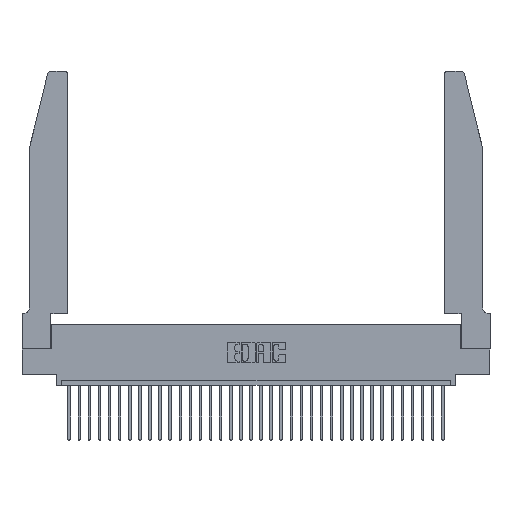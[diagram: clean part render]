
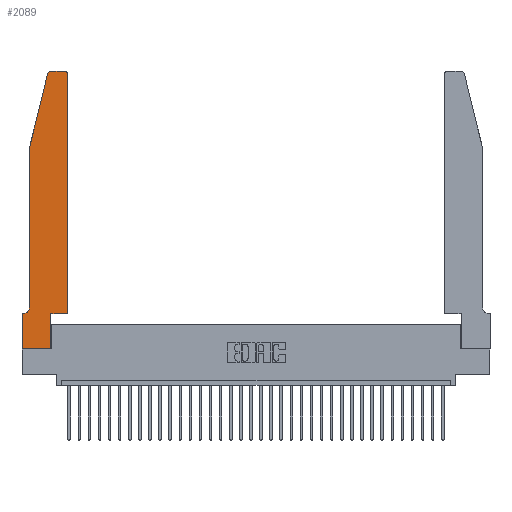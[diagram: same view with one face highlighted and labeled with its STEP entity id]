
A CAD part, top view. The second image highlights one B-rep face of the part: STEP entity #2089.
In plain terms, the highlighted planar face has unit normal (0, 0, 1).
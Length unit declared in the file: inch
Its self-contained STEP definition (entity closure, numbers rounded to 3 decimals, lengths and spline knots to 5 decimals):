
#426 = EDGE_CURVE ( 'NONE', #19606, #13271, #20745, .T. ) ;
#628 = LINE ( 'NONE', #29261, #20833 ) ;
#988 = ORIENTED_EDGE ( 'NONE', *, *, #8348, .T. ) ;
#1811 = ORIENTED_EDGE ( 'NONE', *, *, #30417, .T. ) ;
#2089 = ADVANCED_FACE ( 'NONE', ( #4976 ), #28690, .T. ) ;
#2263 = CARTESIAN_POINT ( 'NONE',  ( 0.4205, 2.75, 0.37 ) ) ;
#2933 = EDGE_CURVE ( 'NONE', #13580, #11461, #31247, .T. ) ;
#3570 = DIRECTION ( 'NONE',  ( 1., 0., 0. ) ) ;
#3638 = ORIENTED_EDGE ( 'NONE', *, *, #2933, .T. ) ;
#4335 = VECTOR ( 'NONE', #23577, 39.37008 ) ;
#4351 = CARTESIAN_POINT ( 'NONE',  ( 0.0755, 2., 0.37 ) ) ;
#4896 = CARTESIAN_POINT ( 'NONE',  ( 0.4205, 2.72, 0.37 ) ) ;
#4976 = FACE_OUTER_BOUND ( 'NONE', #11247, .T. ) ;
#5119 = CARTESIAN_POINT ( 'NONE',  ( 0., 0., 0.37 ) ) ;
#5336 = VECTOR ( 'NONE', #19750, 39.37008 ) ;
#5422 = CARTESIAN_POINT ( 'NONE',  ( 0.284, 2.75, 0.37 ) ) ;
#5726 = VECTOR ( 'NONE', #32244, 39.37008 ) ;
#6444 = CIRCLE ( 'NONE', #33436, 0.07 ) ;
#6450 = EDGE_CURVE ( 'NONE', #32554, #13580, #16539, .T. ) ;
#6557 = LINE ( 'NONE', #13905, #5726 ) ;
#6615 = CARTESIAN_POINT ( 'NONE',  ( 0.0755, 0.42, 0.37 ) ) ;
#7025 = ORIENTED_EDGE ( 'NONE', *, *, #426, .T. ) ;
#7287 = VECTOR ( 'NONE', #32134, 39.37008 ) ;
#7345 = VERTEX_POINT ( 'NONE', #21236 ) ;
#7951 = VERTEX_POINT ( 'NONE', #16158 ) ;
#8083 = EDGE_CURVE ( 'NONE', #18744, #15308, #19302, .T. ) ;
#8348 = EDGE_CURVE ( 'NONE', #11461, #10009, #6557, .T. ) ;
#8799 = CARTESIAN_POINT ( 'NONE',  ( 0., 0., 0.37 ) ) ;
#8819 = ORIENTED_EDGE ( 'NONE', *, *, #29166, .T. ) ;
#8914 = LINE ( 'NONE', #32735, #27896 ) ;
#8915 = CARTESIAN_POINT ( 'NONE',  ( 0., 0., 0.37 ) ) ;
#10009 = VERTEX_POINT ( 'NONE', #6615 ) ;
#10417 = DIRECTION ( 'NONE',  ( -1., 0., 0. ) ) ;
#11015 = VERTEX_POINT ( 'NONE', #5119 ) ;
#11247 = EDGE_LOOP ( 'NONE', ( #8819, #28361, #3638, #988, #25661, #15329, #26457, #33252, #12943, #1811, #26274, #7025 ) ) ;
#11461 = VERTEX_POINT ( 'NONE', #31204 ) ;
#12263 = LINE ( 'NONE', #33175, #17594 ) ;
#12943 = ORIENTED_EDGE ( 'NONE', *, *, #8083, .T. ) ;
#13071 = DIRECTION ( 'NONE',  ( 0., 0., -1. ) ) ;
#13271 = VERTEX_POINT ( 'NONE', #2263 ) ;
#13491 = DIRECTION ( 'NONE',  ( 0., 0., 1. ) ) ;
#13580 = VERTEX_POINT ( 'NONE', #24719 ) ;
#13905 = CARTESIAN_POINT ( 'NONE',  ( 0.0755, 2., 0.37 ) ) ;
#14028 = DIRECTION ( 'NONE',  ( 0., 1., 0. ) ) ;
#14168 = CARTESIAN_POINT ( 'NONE',  ( 0.284, 2.72, 0.37 ) ) ;
#14290 = LINE ( 'NONE', #8799, #7287 ) ;
#15308 = VERTEX_POINT ( 'NONE', #16961 ) ;
#15329 = ORIENTED_EDGE ( 'NONE', *, *, #16720, .T. ) ;
#15502 = DIRECTION ( 'NONE',  ( 1., 0., 0. ) ) ;
#16000 = EDGE_CURVE ( 'NONE', #25353, #11015, #14290, .T. ) ;
#16158 = CARTESIAN_POINT ( 'NONE',  ( 0.0055, 0.35, 0.37 ) ) ;
#16539 = CIRCLE ( 'NONE', #26204, 0.03 ) ;
#16720 = EDGE_CURVE ( 'NONE', #7951, #25353, #628, .T. ) ;
#16961 = CARTESIAN_POINT ( 'NONE',  ( 0.2865, 0.35, 0.37 ) ) ;
#17137 = CARTESIAN_POINT ( 'NONE',  ( 0.2865, 0., 0.37 ) ) ;
#17349 = DIRECTION ( 'NONE',  ( -0.239, -0.971, 0. ) ) ;
#17594 = VECTOR ( 'NONE', #25150, 39.37008 ) ;
#18253 = CARTESIAN_POINT ( 'NONE',  ( 0.0055, 0.42, 0.37 ) ) ;
#18405 = VECTOR ( 'NONE', #29961, 39.37008 ) ;
#18744 = VERTEX_POINT ( 'NONE', #17137 ) ;
#19290 = VECTOR ( 'NONE', #17349, 39.37008 ) ;
#19302 = LINE ( 'NONE', #19627, #5336 ) ;
#19606 = VERTEX_POINT ( 'NONE', #22176 ) ;
#19627 = CARTESIAN_POINT ( 'NONE',  ( 0.2865, 0.35, 0.37 ) ) ;
#19750 = DIRECTION ( 'NONE',  ( 0., 1., 0. ) ) ;
#20395 = EDGE_CURVE ( 'NONE', #7345, #19606, #8914, .T. ) ;
#20745 = CIRCLE ( 'NONE', #29779, 0.03 ) ;
#20833 = VECTOR ( 'NONE', #22249, 39.37008 ) ;
#21236 = CARTESIAN_POINT ( 'NONE',  ( 0.4505, 0.35, 0.37 ) ) ;
#22176 = CARTESIAN_POINT ( 'NONE',  ( 0.4505, 2.72, 0.37 ) ) ;
#22249 = DIRECTION ( 'NONE',  ( -1., 0., 0. ) ) ;
#23577 = DIRECTION ( 'NONE',  ( 1., 0., 0. ) ) ;
#24112 = CARTESIAN_POINT ( 'NONE',  ( 0., 0.35, 0.37 ) ) ;
#24719 = CARTESIAN_POINT ( 'NONE',  ( 0.25487, 2.72718, 0.37 ) ) ;
#25150 = DIRECTION ( 'NONE',  ( -1., 0., 0. ) ) ;
#25353 = VERTEX_POINT ( 'NONE', #24112 ) ;
#25661 = ORIENTED_EDGE ( 'NONE', *, *, #29189, .T. ) ;
#26204 = AXIS2_PLACEMENT_3D ( 'NONE', #14168, #27505, #3570 ) ;
#26274 = ORIENTED_EDGE ( 'NONE', *, *, #20395, .T. ) ;
#26457 = ORIENTED_EDGE ( 'NONE', *, *, #16000, .T. ) ;
#27505 = DIRECTION ( 'NONE',  ( 0., 0., 1. ) ) ;
#27896 = VECTOR ( 'NONE', #14028, 39.37008 ) ;
#28354 = DIRECTION ( 'NONE',  ( 0., 0., 1. ) ) ;
#28361 = ORIENTED_EDGE ( 'NONE', *, *, #6450, .T. ) ;
#28468 = CARTESIAN_POINT ( 'NONE',  ( 0., 0.35, 0.37 ) ) ;
#28499 = AXIS2_PLACEMENT_3D ( 'NONE', #28468, #28354, #15502 ) ;
#28690 = PLANE ( 'NONE',  #28499 ) ;
#28970 = EDGE_CURVE ( 'NONE', #11015, #18744, #32767, .T. ) ;
#29166 = EDGE_CURVE ( 'NONE', #13271, #32554, #12263, .T. ) ;
#29189 = EDGE_CURVE ( 'NONE', #10009, #7951, #6444, .T. ) ;
#29261 = CARTESIAN_POINT ( 'NONE',  ( 0.0755, 0.35, 0.37 ) ) ;
#29779 = AXIS2_PLACEMENT_3D ( 'NONE', #4896, #13491, #31845 ) ;
#29961 = DIRECTION ( 'NONE',  ( 1., 0., 0. ) ) ;
#30417 = EDGE_CURVE ( 'NONE', #15308, #7345, #30648, .T. ) ;
#30648 = LINE ( 'NONE', #33996, #4335 ) ;
#31204 = CARTESIAN_POINT ( 'NONE',  ( 0.0755, 2., 0.37 ) ) ;
#31247 = LINE ( 'NONE', #4351, #19290 ) ;
#31845 = DIRECTION ( 'NONE',  ( 1., 0., 0. ) ) ;
#32134 = DIRECTION ( 'NONE',  ( 0., -1., 0. ) ) ;
#32244 = DIRECTION ( 'NONE',  ( 0., -1., 0. ) ) ;
#32554 = VERTEX_POINT ( 'NONE', #5422 ) ;
#32735 = CARTESIAN_POINT ( 'NONE',  ( 0.4505, 0.35, 0.37 ) ) ;
#32767 = LINE ( 'NONE', #8915, #18405 ) ;
#33175 = CARTESIAN_POINT ( 'NONE',  ( 0.2605, 2.75, 0.37 ) ) ;
#33252 = ORIENTED_EDGE ( 'NONE', *, *, #28970, .T. ) ;
#33436 = AXIS2_PLACEMENT_3D ( 'NONE', #18253, #13071, #10417 ) ;
#33996 = CARTESIAN_POINT ( 'NONE',  ( 0.4505, 0.35, 0.37 ) ) ;
